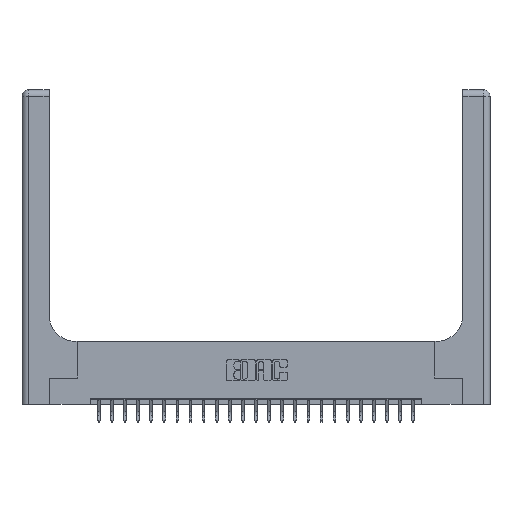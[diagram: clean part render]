
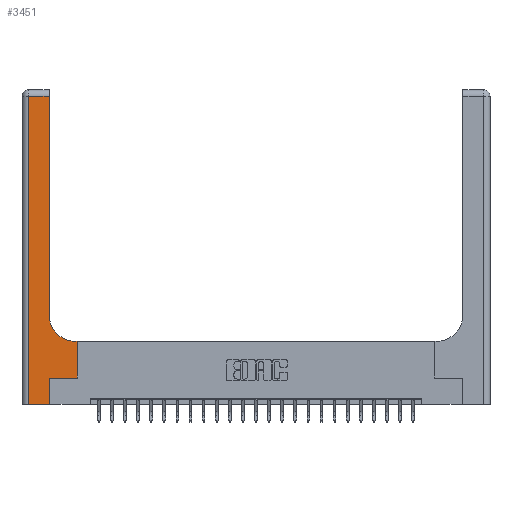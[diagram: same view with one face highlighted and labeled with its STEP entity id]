
A CAD part, top view. The second image highlights one B-rep face of the part: STEP entity #3451.
In plain terms, the highlighted planar face has unit normal (0, 0, 1).
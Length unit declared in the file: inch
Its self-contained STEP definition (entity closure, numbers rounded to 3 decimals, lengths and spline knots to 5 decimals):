
#63 = CARTESIAN_POINT ( 'NONE',  ( 0.528, 0.25, 0.37 ) ) ;
#426 = CARTESIAN_POINT ( 'NONE',  ( 0.265, 0., 0.37 ) ) ;
#705 = CARTESIAN_POINT ( 'NONE',  ( 0.51, 0.85, 0.37 ) ) ;
#1323 = CARTESIAN_POINT ( 'NONE',  ( 0.06, 3., 0.37 ) ) ;
#1648 = DIRECTION ( 'NONE',  ( -1., 0., 0. ) ) ;
#2763 = DIRECTION ( 'NONE',  ( 0., 0., -1. ) ) ;
#2801 = CARTESIAN_POINT ( 'NONE',  ( 0.528, 0.25, 0.37 ) ) ;
#3286 = ORIENTED_EDGE ( 'NONE', *, *, #12339, .T. ) ;
#3307 = LINE ( 'NONE', #3715, #19772 ) ;
#3451 = ADVANCED_FACE ( 'NONE', ( #9897 ), #14944, .F. ) ;
#3459 = CARTESIAN_POINT ( 'NONE',  ( 0.26, 0.6, 0.37 ) ) ;
#3715 = CARTESIAN_POINT ( 'NONE',  ( 0., 2.94, 0.37 ) ) ;
#3976 = VECTOR ( 'NONE', #16922, 39.37008 ) ;
#4581 = EDGE_CURVE ( 'NONE', #10539, #21876, #12965, .T. ) ;
#4774 = VERTEX_POINT ( 'NONE', #14452 ) ;
#4863 = ORIENTED_EDGE ( 'NONE', *, *, #4581, .T. ) ;
#5179 = EDGE_CURVE ( 'NONE', #21530, #6883, #17598, .T. ) ;
#5221 = CARTESIAN_POINT ( 'NONE',  ( 0.51, 0.6, 0.37 ) ) ;
#5718 = ORIENTED_EDGE ( 'NONE', *, *, #14960, .T. ) ;
#6018 = ORIENTED_EDGE ( 'NONE', *, *, #15682, .T. ) ;
#6567 = LINE ( 'NONE', #18683, #3976 ) ;
#6883 = VERTEX_POINT ( 'NONE', #11205 ) ;
#7165 = AXIS2_PLACEMENT_3D ( 'NONE', #19769, #10199, #22916 ) ;
#7358 = CARTESIAN_POINT ( 'NONE',  ( 0.26, 3., 0.37 ) ) ;
#7911 = CARTESIAN_POINT ( 'NONE',  ( 0.265, 0.25, 0.37 ) ) ;
#8087 = VECTOR ( 'NONE', #8250, 39.37008 ) ;
#8165 = EDGE_CURVE ( 'NONE', #12264, #21530, #15165, .T. ) ;
#8250 = DIRECTION ( 'NONE',  ( 0., 1., 0. ) ) ;
#8498 = CARTESIAN_POINT ( 'NONE',  ( 0.26, 0.85, 0.37 ) ) ;
#8986 = VERTEX_POINT ( 'NONE', #63 ) ;
#9184 = VECTOR ( 'NONE', #23772, 39.37008 ) ;
#9402 = DIRECTION ( 'NONE',  ( 0., 1., 0. ) ) ;
#9541 = ORIENTED_EDGE ( 'NONE', *, *, #15590, .T. ) ;
#9897 = FACE_OUTER_BOUND ( 'NONE', #17163, .T. ) ;
#10199 = DIRECTION ( 'NONE',  ( 0., 0., -1. ) ) ;
#10539 = VERTEX_POINT ( 'NONE', #17732 ) ;
#11205 = CARTESIAN_POINT ( 'NONE',  ( 0.26, 2.94, 0.37 ) ) ;
#11360 = ORIENTED_EDGE ( 'NONE', *, *, #8165, .T. ) ;
#11807 = LINE ( 'NONE', #14060, #13530 ) ;
#11952 = CARTESIAN_POINT ( 'NONE',  ( 0.06, 2.94, 0.37 ) ) ;
#12162 = ORIENTED_EDGE ( 'NONE', *, *, #20720, .T. ) ;
#12264 = VERTEX_POINT ( 'NONE', #5221 ) ;
#12339 = EDGE_CURVE ( 'NONE', #4774, #10539, #11807, .T. ) ;
#12662 = VECTOR ( 'NONE', #22169, 39.37008 ) ;
#12965 = LINE ( 'NONE', #426, #8087 ) ;
#13113 = VECTOR ( 'NONE', #16067, 39.37008 ) ;
#13530 = VECTOR ( 'NONE', #19612, 39.37008 ) ;
#14060 = CARTESIAN_POINT ( 'NONE',  ( 0., 0., 0.37 ) ) ;
#14452 = CARTESIAN_POINT ( 'NONE',  ( 0.06, 0., 0.37 ) ) ;
#14558 = LINE ( 'NONE', #2801, #21836 ) ;
#14944 = PLANE ( 'NONE',  #7165 ) ;
#14960 = EDGE_CURVE ( 'NONE', #15570, #12264, #23599, .T. ) ;
#15165 = CIRCLE ( 'NONE', #16056, 0.25 ) ;
#15537 = DIRECTION ( 'NONE',  ( 1., 0., 0. ) ) ;
#15570 = VERTEX_POINT ( 'NONE', #19101 ) ;
#15590 = EDGE_CURVE ( 'NONE', #6883, #19085, #3307, .T. ) ;
#15682 = EDGE_CURVE ( 'NONE', #8986, #15570, #14558, .T. ) ;
#16056 = AXIS2_PLACEMENT_3D ( 'NONE', #705, #2763, #15537 ) ;
#16067 = DIRECTION ( 'NONE',  ( -1., 0., 0. ) ) ;
#16922 = DIRECTION ( 'NONE',  ( 1., 0., 0. ) ) ;
#17163 = EDGE_LOOP ( 'NONE', ( #21358, #9541, #12162, #3286, #4863, #23965, #6018, #5718, #11360 ) ) ;
#17598 = LINE ( 'NONE', #7358, #12662 ) ;
#17732 = CARTESIAN_POINT ( 'NONE',  ( 0.265, 0., 0.37 ) ) ;
#17848 = LINE ( 'NONE', #1323, #9184 ) ;
#18683 = CARTESIAN_POINT ( 'NONE',  ( 0.265, 0.25, 0.37 ) ) ;
#19085 = VERTEX_POINT ( 'NONE', #11952 ) ;
#19101 = CARTESIAN_POINT ( 'NONE',  ( 0.528, 0.6, 0.37 ) ) ;
#19612 = DIRECTION ( 'NONE',  ( 1., 0., 0. ) ) ;
#19769 = CARTESIAN_POINT ( 'NONE',  ( 0., 3., 0.37 ) ) ;
#19772 = VECTOR ( 'NONE', #1648, 39.37008 ) ;
#20235 = EDGE_CURVE ( 'NONE', #21876, #8986, #6567, .T. ) ;
#20720 = EDGE_CURVE ( 'NONE', #19085, #4774, #17848, .T. ) ;
#21358 = ORIENTED_EDGE ( 'NONE', *, *, #5179, .T. ) ;
#21530 = VERTEX_POINT ( 'NONE', #8498 ) ;
#21836 = VECTOR ( 'NONE', #9402, 39.37008 ) ;
#21876 = VERTEX_POINT ( 'NONE', #7911 ) ;
#22169 = DIRECTION ( 'NONE',  ( 0., 1., 0. ) ) ;
#22916 = DIRECTION ( 'NONE',  ( -1., 0., 0. ) ) ;
#23599 = LINE ( 'NONE', #3459, #13113 ) ;
#23772 = DIRECTION ( 'NONE',  ( 0., -1., 0. ) ) ;
#23965 = ORIENTED_EDGE ( 'NONE', *, *, #20235, .T. ) ;
